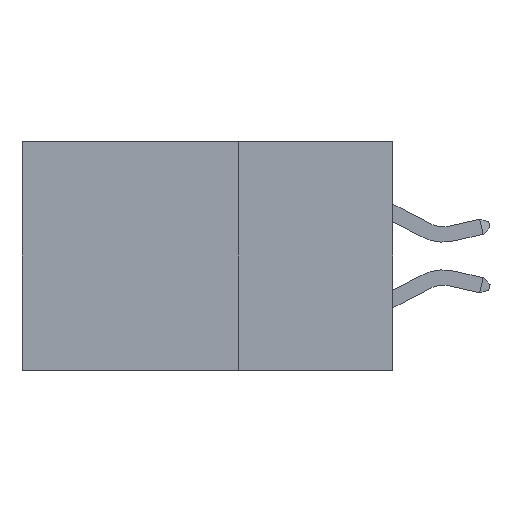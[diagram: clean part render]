
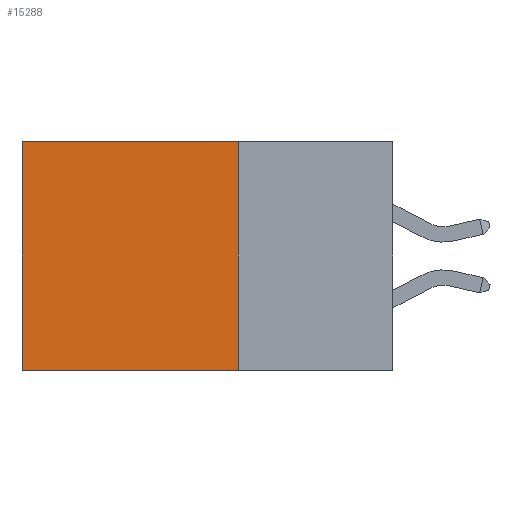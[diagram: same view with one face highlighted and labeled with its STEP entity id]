
A CAD part, left-side view. The second image highlights one B-rep face of the part: STEP entity #15288.
In plain terms, the highlighted planar face has unit normal (-1, 0, 0).
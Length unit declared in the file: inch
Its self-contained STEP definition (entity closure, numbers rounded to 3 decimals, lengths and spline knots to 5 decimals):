
#225 = VERTEX_POINT ( 'NONE', #2734 ) ;
#791 = DIRECTION ( 'NONE',  ( 0., 0., -1. ) ) ;
#1955 = DIRECTION ( 'NONE',  ( 0., 0., -1. ) ) ;
#2010 = CARTESIAN_POINT ( 'NONE',  ( 0.2875, 0.25, 0. ) ) ;
#2176 = VERTEX_POINT ( 'NONE', #19579 ) ;
#2734 = CARTESIAN_POINT ( 'NONE',  ( 0.2875, 0.25, -0.37 ) ) ;
#3703 = EDGE_CURVE ( 'NONE', #20806, #225, #4480, .T. ) ;
#4304 = LINE ( 'NONE', #17957, #17720 ) ;
#4480 = LINE ( 'NONE', #2010, #13383 ) ;
#5352 = EDGE_CURVE ( 'NONE', #225, #2176, #20131, .T. ) ;
#5584 = FACE_OUTER_BOUND ( 'NONE', #8203, .T. ) ;
#6830 = AXIS2_PLACEMENT_3D ( 'NONE', #12230, #17443, #7009 ) ;
#7009 = DIRECTION ( 'NONE',  ( 0., 0., -1. ) ) ;
#8203 = EDGE_LOOP ( 'NONE', ( #14648, #14731, #19771, #22078 ) ) ;
#10896 = EDGE_CURVE ( 'NONE', #17645, #2176, #21140, .T. ) ;
#12161 = VECTOR ( 'NONE', #791, 39.37008 ) ;
#12230 = CARTESIAN_POINT ( 'NONE',  ( 0.2875, 0.25, 0. ) ) ;
#12727 = EDGE_CURVE ( 'NONE', #20806, #17645, #4304, .T. ) ;
#13383 = VECTOR ( 'NONE', #1955, 39.37008 ) ;
#14013 = CARTESIAN_POINT ( 'NONE',  ( 0.2875, 0.25, -0.37 ) ) ;
#14024 = PLANE ( 'NONE',  #6830 ) ;
#14648 = ORIENTED_EDGE ( 'NONE', *, *, #10896, .T. ) ;
#14654 = DIRECTION ( 'NONE',  ( 0., 1., 0. ) ) ;
#14731 = ORIENTED_EDGE ( 'NONE', *, *, #5352, .F. ) ;
#14870 = CARTESIAN_POINT ( 'NONE',  ( 0.2875, 0.25, 0. ) ) ;
#15288 = ADVANCED_FACE ( 'NONE', ( #5584 ), #14024, .F. ) ;
#15703 = VECTOR ( 'NONE', #22402, 39.37008 ) ;
#16816 = CARTESIAN_POINT ( 'NONE',  ( 0.2875, 0.6, 0. ) ) ;
#17443 = DIRECTION ( 'NONE',  ( 1., 0., 0. ) ) ;
#17645 = VERTEX_POINT ( 'NONE', #20798 ) ;
#17720 = VECTOR ( 'NONE', #14654, 39.37008 ) ;
#17957 = CARTESIAN_POINT ( 'NONE',  ( 0.2875, 0.25, 0. ) ) ;
#19579 = CARTESIAN_POINT ( 'NONE',  ( 0.2875, 0.6, -0.37 ) ) ;
#19771 = ORIENTED_EDGE ( 'NONE', *, *, #3703, .F. ) ;
#20131 = LINE ( 'NONE', #14013, #15703 ) ;
#20798 = CARTESIAN_POINT ( 'NONE',  ( 0.2875, 0.6, 0. ) ) ;
#20806 = VERTEX_POINT ( 'NONE', #14870 ) ;
#21140 = LINE ( 'NONE', #16816, #12161 ) ;
#22078 = ORIENTED_EDGE ( 'NONE', *, *, #12727, .T. ) ;
#22402 = DIRECTION ( 'NONE',  ( 0., 1., 0. ) ) ;
